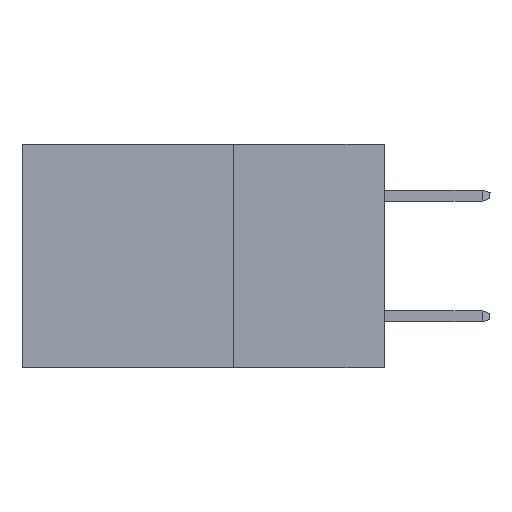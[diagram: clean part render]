
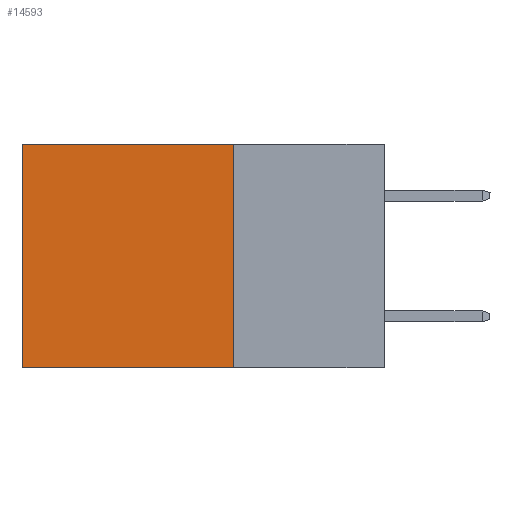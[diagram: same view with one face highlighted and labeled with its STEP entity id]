
A CAD part, left-side view. The second image highlights one B-rep face of the part: STEP entity #14593.
In plain terms, the highlighted planar face has unit normal (-1, 0, 0).
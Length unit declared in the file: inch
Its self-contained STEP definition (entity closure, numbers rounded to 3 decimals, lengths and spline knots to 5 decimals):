
#6232 = LINE ( 'NONE', #25473, #26010 ) ;
#6675 = CARTESIAN_POINT ( 'NONE',  ( 0.2615, 0.25, -0.37 ) ) ;
#6761 = EDGE_CURVE ( 'NONE', #16234, #19175, #9045, .T. ) ;
#6935 = VERTEX_POINT ( 'NONE', #20682 ) ;
#7763 = LINE ( 'NONE', #6675, #17949 ) ;
#8750 = DIRECTION ( 'NONE',  ( 0., 0., -1. ) ) ;
#9045 = LINE ( 'NONE', #20259, #13818 ) ;
#9159 = CARTESIAN_POINT ( 'NONE',  ( 0.2615, 0.25, -0.37 ) ) ;
#9162 = EDGE_CURVE ( 'NONE', #6935, #19175, #26103, .T. ) ;
#9887 = VECTOR ( 'NONE', #11202, 39.37008 ) ;
#10500 = CARTESIAN_POINT ( 'NONE',  ( 0.2615, 0.6, 0. ) ) ;
#10903 = CARTESIAN_POINT ( 'NONE',  ( 0.2615, 0.25, -0.37 ) ) ;
#11202 = DIRECTION ( 'NONE',  ( 0., 1., 0. ) ) ;
#11959 = EDGE_LOOP ( 'NONE', ( #13446, #12719, #21162, #21097 ) ) ;
#11972 = FACE_OUTER_BOUND ( 'NONE', #11959, .T. ) ;
#12719 = ORIENTED_EDGE ( 'NONE', *, *, #9162, .F. ) ;
#12952 = DIRECTION ( 'NONE',  ( 0., 0., -1. ) ) ;
#13339 = EDGE_CURVE ( 'NONE', #15632, #16234, #6232, .T. ) ;
#13446 = ORIENTED_EDGE ( 'NONE', *, *, #6761, .T. ) ;
#13818 = VECTOR ( 'NONE', #14142, 39.37008 ) ;
#14142 = DIRECTION ( 'NONE',  ( 0., 0., -1. ) ) ;
#14394 = AXIS2_PLACEMENT_3D ( 'NONE', #10903, #25147, #12952 ) ;
#14593 = ADVANCED_FACE ( 'NONE', ( #11972 ), #23066, .F. ) ;
#15308 = DIRECTION ( 'NONE',  ( 0., 1., 0. ) ) ;
#15632 = VERTEX_POINT ( 'NONE', #18602 ) ;
#16234 = VERTEX_POINT ( 'NONE', #10500 ) ;
#17949 = VECTOR ( 'NONE', #8750, 39.37008 ) ;
#18602 = CARTESIAN_POINT ( 'NONE',  ( 0.2615, 0.25, 0. ) ) ;
#18688 = EDGE_CURVE ( 'NONE', #15632, #6935, #7763, .T. ) ;
#19175 = VERTEX_POINT ( 'NONE', #20277 ) ;
#20259 = CARTESIAN_POINT ( 'NONE',  ( 0.2615, 0.6, -0.37 ) ) ;
#20277 = CARTESIAN_POINT ( 'NONE',  ( 0.2615, 0.6, -0.37 ) ) ;
#20682 = CARTESIAN_POINT ( 'NONE',  ( 0.2615, 0.25, -0.37 ) ) ;
#21097 = ORIENTED_EDGE ( 'NONE', *, *, #13339, .T. ) ;
#21162 = ORIENTED_EDGE ( 'NONE', *, *, #18688, .F. ) ;
#23066 = PLANE ( 'NONE',  #14394 ) ;
#25147 = DIRECTION ( 'NONE',  ( 1., 0., 0. ) ) ;
#25473 = CARTESIAN_POINT ( 'NONE',  ( 0.2615, 0.25, 0. ) ) ;
#26010 = VECTOR ( 'NONE', #15308, 39.37008 ) ;
#26103 = LINE ( 'NONE', #9159, #9887 ) ;
